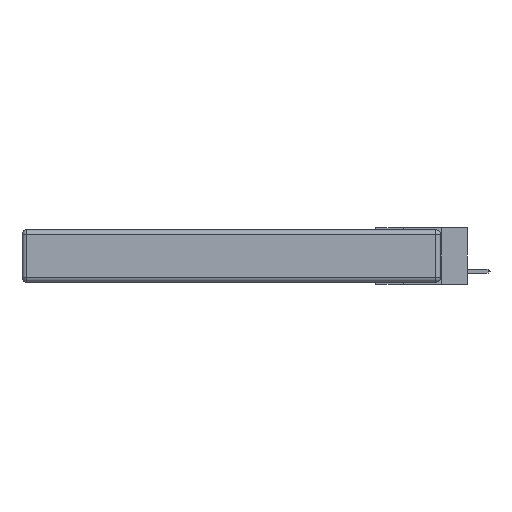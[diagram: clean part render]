
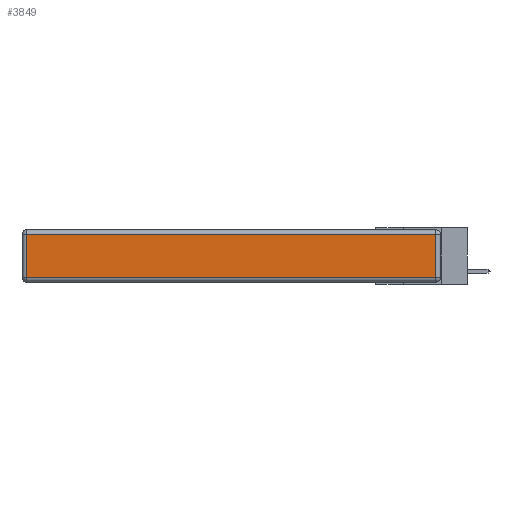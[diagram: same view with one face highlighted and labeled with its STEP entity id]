
A CAD part, left-side view. The second image highlights one B-rep face of the part: STEP entity #3849.
In plain terms, the highlighted planar face has unit normal (-1, 0, 0).
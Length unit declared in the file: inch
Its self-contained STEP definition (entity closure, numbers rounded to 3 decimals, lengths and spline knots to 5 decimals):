
#676 = ORIENTED_EDGE ( 'NONE', *, *, #13140, .T. ) ;
#897 = CARTESIAN_POINT ( 'NONE',  ( 0., 2.72, -0.03 ) ) ;
#1202 = VECTOR ( 'NONE', #1990, 39.37008 ) ;
#1940 = CARTESIAN_POINT ( 'NONE',  ( 0., 0., -0.313 ) ) ;
#1981 = EDGE_CURVE ( 'NONE', #5516, #4512, #10860, .T. ) ;
#1990 = DIRECTION ( 'NONE',  ( 0., -1., 0. ) ) ;
#2559 = ORIENTED_EDGE ( 'NONE', *, *, #13288, .T. ) ;
#3223 = VECTOR ( 'NONE', #4186, 39.37008 ) ;
#3849 = ADVANCED_FACE ( 'NONE', ( #11884 ), #5208, .T. ) ;
#3935 = LINE ( 'NONE', #13092, #4893 ) ;
#4186 = DIRECTION ( 'NONE',  ( 0., 0., -1. ) ) ;
#4512 = VERTEX_POINT ( 'NONE', #10719 ) ;
#4669 = DIRECTION ( 'NONE',  ( 0., 1., 0. ) ) ;
#4893 = VECTOR ( 'NONE', #4669, 39.37008 ) ;
#4997 = VERTEX_POINT ( 'NONE', #897 ) ;
#5208 = PLANE ( 'NONE',  #8372 ) ;
#5516 = VERTEX_POINT ( 'NONE', #10155 ) ;
#6595 = VERTEX_POINT ( 'NONE', #14217 ) ;
#8372 = AXIS2_PLACEMENT_3D ( 'NONE', #10274, #10174, #11449 ) ;
#8515 = EDGE_LOOP ( 'NONE', ( #13595, #676, #8901, #2559 ) ) ;
#8579 = VECTOR ( 'NONE', #12151, 39.37008 ) ;
#8901 = ORIENTED_EDGE ( 'NONE', *, *, #13860, .T. ) ;
#10155 = CARTESIAN_POINT ( 'NONE',  ( 0., 2.72, -0.313 ) ) ;
#10174 = DIRECTION ( 'NONE',  ( -1., 0., 0. ) ) ;
#10274 = CARTESIAN_POINT ( 'NONE',  ( 0., 0., -0.343 ) ) ;
#10719 = CARTESIAN_POINT ( 'NONE',  ( 0., 0.03, -0.313 ) ) ;
#10860 = LINE ( 'NONE', #1940, #1202 ) ;
#11449 = DIRECTION ( 'NONE',  ( 0., 0., 1. ) ) ;
#11884 = FACE_OUTER_BOUND ( 'NONE', #8515, .T. ) ;
#12151 = DIRECTION ( 'NONE',  ( 0., 0., 1. ) ) ;
#12272 = LINE ( 'NONE', #13343, #8579 ) ;
#13066 = LINE ( 'NONE', #13781, #3223 ) ;
#13092 = CARTESIAN_POINT ( 'NONE',  ( 0., 2.75, -0.03 ) ) ;
#13140 = EDGE_CURVE ( 'NONE', #4512, #6595, #12272, .T. ) ;
#13288 = EDGE_CURVE ( 'NONE', #4997, #5516, #13066, .T. ) ;
#13343 = CARTESIAN_POINT ( 'NONE',  ( 0., 0.03, -0.343 ) ) ;
#13595 = ORIENTED_EDGE ( 'NONE', *, *, #1981, .T. ) ;
#13781 = CARTESIAN_POINT ( 'NONE',  ( 0., 2.72, -0.343 ) ) ;
#13860 = EDGE_CURVE ( 'NONE', #6595, #4997, #3935, .T. ) ;
#14217 = CARTESIAN_POINT ( 'NONE',  ( 0., 0.03, -0.03 ) ) ;
